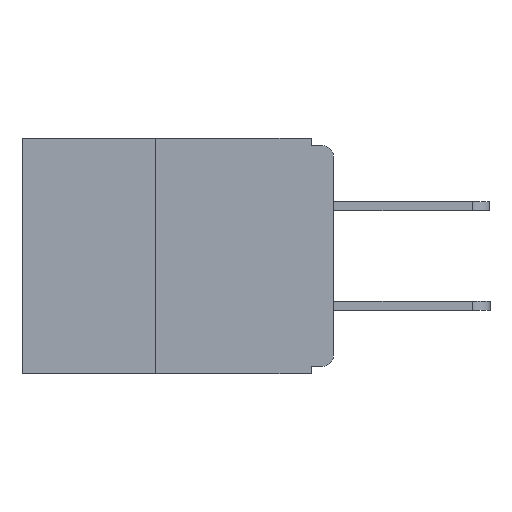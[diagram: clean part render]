
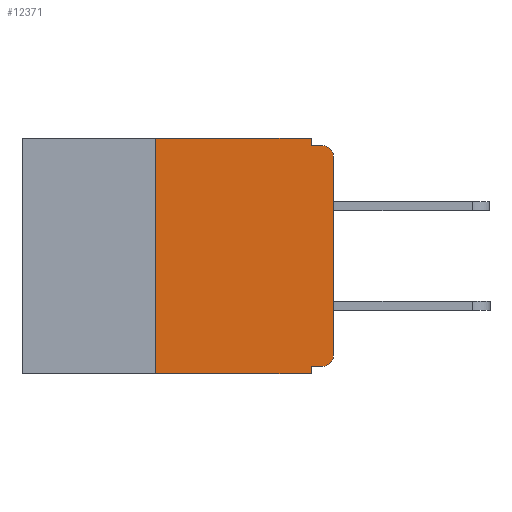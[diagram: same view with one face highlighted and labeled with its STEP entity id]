
A CAD part, left-side view. The second image highlights one B-rep face of the part: STEP entity #12371.
In plain terms, the highlighted planar face has unit normal (-1, 0, 0).
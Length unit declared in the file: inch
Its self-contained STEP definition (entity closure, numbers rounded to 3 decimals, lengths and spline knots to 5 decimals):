
#395 = VERTEX_POINT ( 'NONE', #9514 ) ;
#632 = ORIENTED_EDGE ( 'NONE', *, *, #1668, .T. ) ;
#986 = VECTOR ( 'NONE', #10644, 39.37008 ) ;
#1039 = LINE ( 'NONE', #15044, #13590 ) ;
#1668 = EDGE_CURVE ( 'NONE', #4169, #15115, #1039, .T. ) ;
#2069 = PLANE ( 'NONE',  #20007 ) ;
#3078 = EDGE_LOOP ( 'NONE', ( #15082, #15822, #14100, #4763, #4329, #5402, #632, #17824, #3828, #14371 ) ) ;
#3169 = EDGE_CURVE ( 'NONE', #14703, #9225, #15246, .T. ) ;
#3287 = VECTOR ( 'NONE', #15632, 39.37008 ) ;
#3828 = ORIENTED_EDGE ( 'NONE', *, *, #11609, .F. ) ;
#3834 = LINE ( 'NONE', #18646, #3287 ) ;
#3947 = EDGE_CURVE ( 'NONE', #3974, #15115, #10268, .T. ) ;
#3974 = VERTEX_POINT ( 'NONE', #18460 ) ;
#4073 = EDGE_CURVE ( 'NONE', #17405, #9225, #16604, .T. ) ;
#4169 = VERTEX_POINT ( 'NONE', #16599 ) ;
#4329 = ORIENTED_EDGE ( 'NONE', *, *, #15894, .F. ) ;
#4763 = ORIENTED_EDGE ( 'NONE', *, *, #20265, .F. ) ;
#5076 = CARTESIAN_POINT ( 'NONE',  ( 0., 0.031, -0.33 ) ) ;
#5087 = LINE ( 'NONE', #15152, #13177 ) ;
#5402 = ORIENTED_EDGE ( 'NONE', *, *, #17204, .F. ) ;
#5464 = CARTESIAN_POINT ( 'NONE',  ( 0., 0.437, 0. ) ) ;
#5914 = VECTOR ( 'NONE', #19130, 39.37008 ) ;
#6563 = CARTESIAN_POINT ( 'NONE',  ( 0., 0.015, -0.32 ) ) ;
#7041 = CARTESIAN_POINT ( 'NONE',  ( 0., 0.015, -0.305 ) ) ;
#7730 = VERTEX_POINT ( 'NONE', #6563 ) ;
#8173 = CARTESIAN_POINT ( 'NONE',  ( 0., 0., 0. ) ) ;
#8352 = EDGE_CURVE ( 'NONE', #13387, #17405, #10587, .T. ) ;
#8632 = AXIS2_PLACEMENT_3D ( 'NONE', #17567, #17545, #17517 ) ;
#8684 = DIRECTION ( 'NONE',  ( 0., 0., -1. ) ) ;
#8779 = DIRECTION ( 'NONE',  ( 1., 0., 0. ) ) ;
#9225 = VERTEX_POINT ( 'NONE', #16212 ) ;
#9514 = CARTESIAN_POINT ( 'NONE',  ( 0., 0.031, 0. ) ) ;
#10090 = CARTESIAN_POINT ( 'NONE',  ( 0., 0., -0.305 ) ) ;
#10268 = LINE ( 'NONE', #18980, #5914 ) ;
#10394 = CARTESIAN_POINT ( 'NONE',  ( 0., 0.25, 0. ) ) ;
#10587 = LINE ( 'NONE', #8173, #18379 ) ;
#10644 = DIRECTION ( 'NONE',  ( 0., 0., -1. ) ) ;
#11609 = EDGE_CURVE ( 'NONE', #7730, #3974, #12625, .T. ) ;
#11680 = CARTESIAN_POINT ( 'NONE',  ( 0., 0.031, -0.01 ) ) ;
#12196 = CARTESIAN_POINT ( 'NONE',  ( 0., 0.031, 0. ) ) ;
#12371 = ADVANCED_FACE ( 'NONE', ( #15487 ), #2069, .F. ) ;
#12386 = VERTEX_POINT ( 'NONE', #10394 ) ;
#12625 = LINE ( 'NONE', #17559, #16243 ) ;
#12939 = DIRECTION ( 'NONE',  ( 0., 1., 0. ) ) ;
#13177 = VECTOR ( 'NONE', #16700, 39.37008 ) ;
#13387 = VERTEX_POINT ( 'NONE', #10090 ) ;
#13590 = VECTOR ( 'NONE', #16749, 39.37008 ) ;
#14100 = ORIENTED_EDGE ( 'NONE', *, *, #3169, .F. ) ;
#14371 = ORIENTED_EDGE ( 'NONE', *, *, #18866, .T. ) ;
#14703 = VERTEX_POINT ( 'NONE', #11680 ) ;
#15044 = CARTESIAN_POINT ( 'NONE',  ( 0., 0.437, -0.33 ) ) ;
#15082 = ORIENTED_EDGE ( 'NONE', *, *, #8352, .T. ) ;
#15115 = VERTEX_POINT ( 'NONE', #5076 ) ;
#15152 = CARTESIAN_POINT ( 'NONE',  ( 0., 0.437, 0. ) ) ;
#15246 = LINE ( 'NONE', #19792, #19311 ) ;
#15487 = FACE_OUTER_BOUND ( 'NONE', #3078, .T. ) ;
#15632 = DIRECTION ( 'NONE',  ( 0., 0., 1. ) ) ;
#15822 = ORIENTED_EDGE ( 'NONE', *, *, #4073, .T. ) ;
#15894 = EDGE_CURVE ( 'NONE', #12386, #395, #5087, .T. ) ;
#16212 = CARTESIAN_POINT ( 'NONE',  ( 0., 0.015, -0.01 ) ) ;
#16243 = VECTOR ( 'NONE', #12939, 39.37008 ) ;
#16379 = AXIS2_PLACEMENT_3D ( 'NONE', #7041, #18071, #8684 ) ;
#16525 = CIRCLE ( 'NONE', #16379, 0.015 ) ;
#16599 = CARTESIAN_POINT ( 'NONE',  ( 0., 0.25, -0.33 ) ) ;
#16604 = CIRCLE ( 'NONE', #8632, 0.015 ) ;
#16700 = DIRECTION ( 'NONE',  ( 0., -1., 0. ) ) ;
#16749 = DIRECTION ( 'NONE',  ( 0., -1., 0. ) ) ;
#17204 = EDGE_CURVE ( 'NONE', #4169, #12386, #3834, .T. ) ;
#17405 = VERTEX_POINT ( 'NONE', #20633 ) ;
#17517 = DIRECTION ( 'NONE',  ( 0., 0., -1. ) ) ;
#17545 = DIRECTION ( 'NONE',  ( -1., 0., 0. ) ) ;
#17559 = CARTESIAN_POINT ( 'NONE',  ( 0., 0., -0.32 ) ) ;
#17567 = CARTESIAN_POINT ( 'NONE',  ( 0., 0.015, -0.025 ) ) ;
#17824 = ORIENTED_EDGE ( 'NONE', *, *, #3947, .F. ) ;
#18071 = DIRECTION ( 'NONE',  ( -1., 0., 0. ) ) ;
#18160 = LINE ( 'NONE', #12196, #986 ) ;
#18379 = VECTOR ( 'NONE', #20649, 39.37008 ) ;
#18460 = CARTESIAN_POINT ( 'NONE',  ( 0., 0.031, -0.32 ) ) ;
#18646 = CARTESIAN_POINT ( 'NONE',  ( 0., 0.25, -0.33 ) ) ;
#18866 = EDGE_CURVE ( 'NONE', #7730, #13387, #16525, .T. ) ;
#18980 = CARTESIAN_POINT ( 'NONE',  ( 0., 0.031, -0.33 ) ) ;
#19130 = DIRECTION ( 'NONE',  ( 0., 0., -1. ) ) ;
#19311 = VECTOR ( 'NONE', #19532, 39.37008 ) ;
#19532 = DIRECTION ( 'NONE',  ( 0., -1., 0. ) ) ;
#19661 = DIRECTION ( 'NONE',  ( 0., 0., -1. ) ) ;
#19792 = CARTESIAN_POINT ( 'NONE',  ( 0., 0., -0.01 ) ) ;
#20007 = AXIS2_PLACEMENT_3D ( 'NONE', #5464, #8779, #19661 ) ;
#20265 = EDGE_CURVE ( 'NONE', #395, #14703, #18160, .T. ) ;
#20633 = CARTESIAN_POINT ( 'NONE',  ( 0., 0., -0.025 ) ) ;
#20649 = DIRECTION ( 'NONE',  ( 0., 0., 1. ) ) ;
